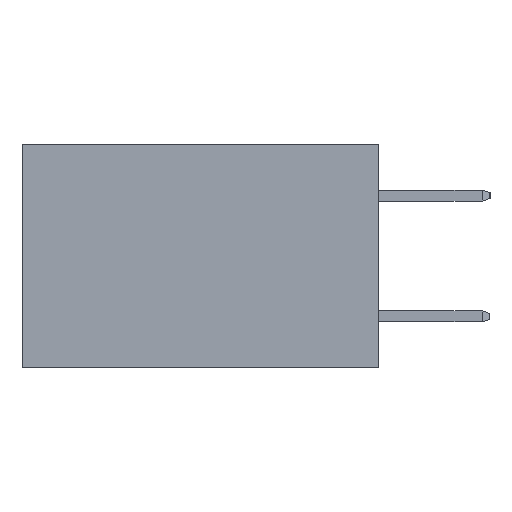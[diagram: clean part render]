
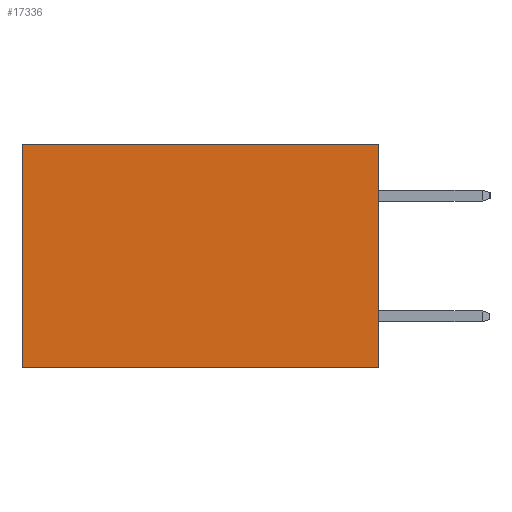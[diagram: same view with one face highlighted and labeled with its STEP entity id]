
A CAD part, left-side view. The second image highlights one B-rep face of the part: STEP entity #17336.
In plain terms, the highlighted planar face has unit normal (-1, 0, 0).
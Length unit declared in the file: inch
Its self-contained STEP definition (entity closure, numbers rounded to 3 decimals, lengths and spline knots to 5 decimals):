
#10 = CARTESIAN_POINT ( 'NONE',  ( 0.277, 0.59, 0. ) ) ;
#1083 = VECTOR ( 'NONE', #15405, 39.37008 ) ;
#1152 = VERTEX_POINT ( 'NONE', #10 ) ;
#1305 = CARTESIAN_POINT ( 'NONE',  ( 0.277, 0.59, -0.37 ) ) ;
#1536 = ORIENTED_EDGE ( 'NONE', *, *, #6594, .F. ) ;
#1601 = DIRECTION ( 'NONE',  ( 0., 0., -1. ) ) ;
#1707 = EDGE_CURVE ( 'NONE', #10559, #22165, #19769, .T. ) ;
#3176 = ORIENTED_EDGE ( 'NONE', *, *, #1707, .F. ) ;
#3284 = VERTEX_POINT ( 'NONE', #6480 ) ;
#3560 = VECTOR ( 'NONE', #11423, 39.37008 ) ;
#4618 = CARTESIAN_POINT ( 'NONE',  ( 0.277, 0., -0.37 ) ) ;
#5107 = CARTESIAN_POINT ( 'NONE',  ( 0.277, 0., -0.37 ) ) ;
#6480 = CARTESIAN_POINT ( 'NONE',  ( 0.277, 0., 0. ) ) ;
#6594 = EDGE_CURVE ( 'NONE', #3284, #10559, #13669, .T. ) ;
#6800 = FACE_OUTER_BOUND ( 'NONE', #7513, .T. ) ;
#7513 = EDGE_LOOP ( 'NONE', ( #7953, #3176, #1536, #11343 ) ) ;
#7953 = ORIENTED_EDGE ( 'NONE', *, *, #19011, .T. ) ;
#8208 = CARTESIAN_POINT ( 'NONE',  ( 0.277, 0.59, -0.37 ) ) ;
#9841 = DIRECTION ( 'NONE',  ( 0., 1., 0. ) ) ;
#10559 = VERTEX_POINT ( 'NONE', #5107 ) ;
#10590 = PLANE ( 'NONE',  #16999 ) ;
#10659 = LINE ( 'NONE', #8208, #1083 ) ;
#11343 = ORIENTED_EDGE ( 'NONE', *, *, #13585, .T. ) ;
#11423 = DIRECTION ( 'NONE',  ( 0., 0., -1. ) ) ;
#11602 = CARTESIAN_POINT ( 'NONE',  ( 0.277, 0., -0.37 ) ) ;
#12367 = DIRECTION ( 'NONE',  ( 1., 0., 0. ) ) ;
#12983 = CARTESIAN_POINT ( 'NONE',  ( 0.277, 0., 0. ) ) ;
#13585 = EDGE_CURVE ( 'NONE', #3284, #1152, #18759, .T. ) ;
#13669 = LINE ( 'NONE', #11602, #3560 ) ;
#14773 = DIRECTION ( 'NONE',  ( 0., 1., 0. ) ) ;
#15065 = VECTOR ( 'NONE', #9841, 39.37008 ) ;
#15405 = DIRECTION ( 'NONE',  ( 0., 0., -1. ) ) ;
#16999 = AXIS2_PLACEMENT_3D ( 'NONE', #22959, #12367, #1601 ) ;
#17336 = ADVANCED_FACE ( 'NONE', ( #6800 ), #10590, .F. ) ;
#17658 = VECTOR ( 'NONE', #14773, 39.37008 ) ;
#18759 = LINE ( 'NONE', #12983, #17658 ) ;
#19011 = EDGE_CURVE ( 'NONE', #1152, #22165, #10659, .T. ) ;
#19769 = LINE ( 'NONE', #4618, #15065 ) ;
#22165 = VERTEX_POINT ( 'NONE', #1305 ) ;
#22959 = CARTESIAN_POINT ( 'NONE',  ( 0.277, 0., -0.37 ) ) ;
